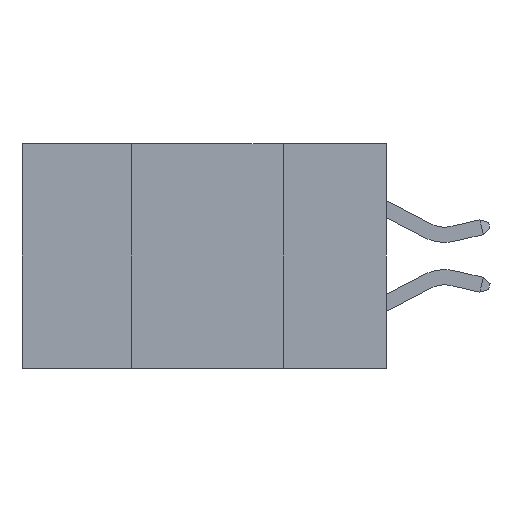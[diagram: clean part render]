
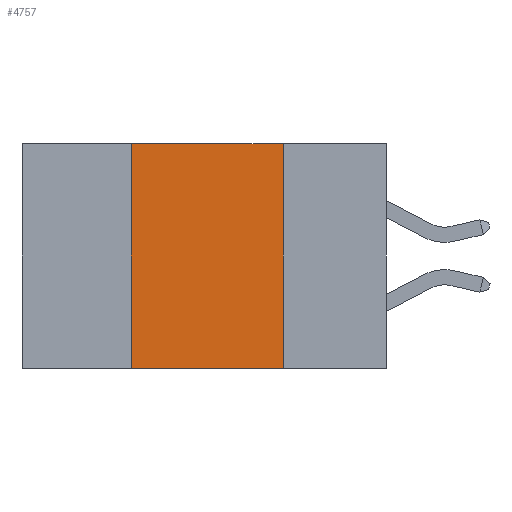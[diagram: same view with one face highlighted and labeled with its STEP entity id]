
A CAD part, left-side view. The second image highlights one B-rep face of the part: STEP entity #4757.
In plain terms, the highlighted planar face has unit normal (-1, 0, 0).
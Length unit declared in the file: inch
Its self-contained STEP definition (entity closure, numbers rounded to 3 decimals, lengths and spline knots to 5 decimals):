
#732 = CARTESIAN_POINT ( 'NONE',  ( 0., 0.42, 0. ) ) ;
#865 = EDGE_LOOP ( 'NONE', ( #5109, #6131, #20105, #24320 ) ) ;
#1701 = VERTEX_POINT ( 'NONE', #2413 ) ;
#2379 = FACE_OUTER_BOUND ( 'NONE', #865, .T. ) ;
#2413 = CARTESIAN_POINT ( 'NONE',  ( 0., 0.17, 0. ) ) ;
#2467 = PLANE ( 'NONE',  #16768 ) ;
#2491 = DIRECTION ( 'NONE',  ( 0., 0., -1. ) ) ;
#2529 = EDGE_CURVE ( 'NONE', #16827, #7466, #3643, .T. ) ;
#2876 = DIRECTION ( 'NONE',  ( 0., -1., 0. ) ) ;
#3643 = LINE ( 'NONE', #16152, #10479 ) ;
#4757 = ADVANCED_FACE ( 'NONE', ( #2379 ), #2467, .F. ) ;
#5109 = ORIENTED_EDGE ( 'NONE', *, *, #5789, .F. ) ;
#5789 = EDGE_CURVE ( 'NONE', #1701, #6333, #7355, .T. ) ;
#6128 = CARTESIAN_POINT ( 'NONE',  ( 0., 0.6, 0. ) ) ;
#6131 = ORIENTED_EDGE ( 'NONE', *, *, #17844, .F. ) ;
#6333 = VERTEX_POINT ( 'NONE', #17418 ) ;
#6835 = EDGE_CURVE ( 'NONE', #16827, #6333, #13508, .T. ) ;
#7355 = LINE ( 'NONE', #23916, #11203 ) ;
#7466 = VERTEX_POINT ( 'NONE', #732 ) ;
#10023 = DIRECTION ( 'NONE',  ( 0., 0., -1. ) ) ;
#10479 = VECTOR ( 'NONE', #21977, 39.37008 ) ;
#11203 = VECTOR ( 'NONE', #2491, 39.37008 ) ;
#11428 = DIRECTION ( 'NONE',  ( 0., -1., 0. ) ) ;
#13508 = LINE ( 'NONE', #14241, #20295 ) ;
#14241 = CARTESIAN_POINT ( 'NONE',  ( 0., 0.6, -0.37 ) ) ;
#14368 = VECTOR ( 'NONE', #11428, 39.37008 ) ;
#16152 = CARTESIAN_POINT ( 'NONE',  ( 0., 0.42, 0. ) ) ;
#16768 = AXIS2_PLACEMENT_3D ( 'NONE', #6128, #23089, #10023 ) ;
#16827 = VERTEX_POINT ( 'NONE', #23741 ) ;
#17270 = CARTESIAN_POINT ( 'NONE',  ( 0., 0.6, 0. ) ) ;
#17418 = CARTESIAN_POINT ( 'NONE',  ( 0., 0.17, -0.37 ) ) ;
#17844 = EDGE_CURVE ( 'NONE', #7466, #1701, #22635, .T. ) ;
#20105 = ORIENTED_EDGE ( 'NONE', *, *, #2529, .F. ) ;
#20295 = VECTOR ( 'NONE', #2876, 39.37008 ) ;
#21977 = DIRECTION ( 'NONE',  ( 0., 0., 1. ) ) ;
#22635 = LINE ( 'NONE', #17270, #14368 ) ;
#23089 = DIRECTION ( 'NONE',  ( 1., 0., 0. ) ) ;
#23741 = CARTESIAN_POINT ( 'NONE',  ( 0., 0.42, -0.37 ) ) ;
#23916 = CARTESIAN_POINT ( 'NONE',  ( 0., 0.17, 0. ) ) ;
#24320 = ORIENTED_EDGE ( 'NONE', *, *, #6835, .T. ) ;
